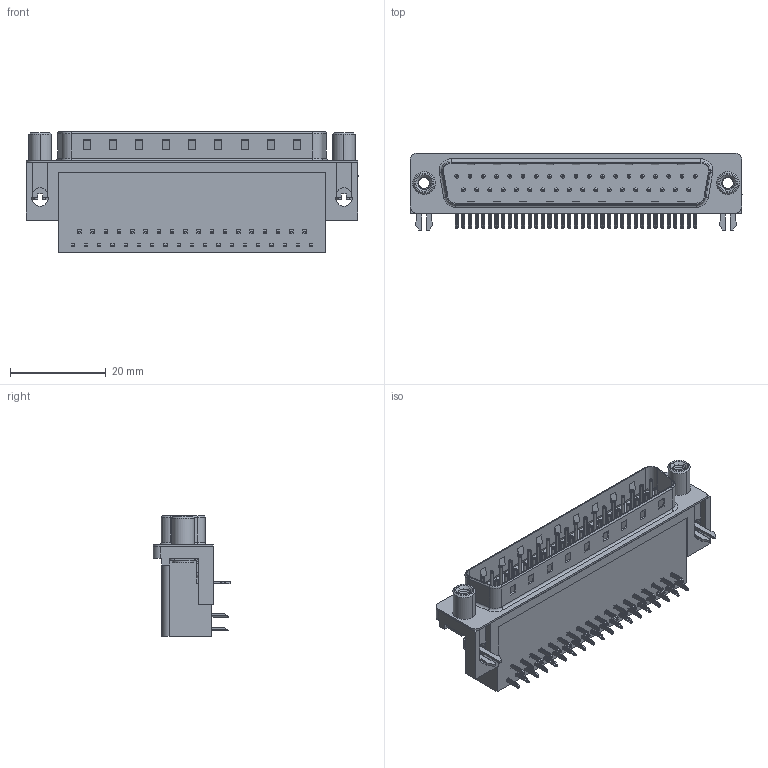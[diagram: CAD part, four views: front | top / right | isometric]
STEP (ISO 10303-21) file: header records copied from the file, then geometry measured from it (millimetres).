
FILE_DESCRIPTION (( 'STEP AP203' ), '1' );
FILE_NAME ('625-037-362-530.STEP', '2018-11-06T05:58:14', ( '' ), ( '' ), 'SwSTEP 2.0', 'SolidWorks 2016', '' );
FILE_SCHEMA (( 'CONFIG_CONTROL_DESIGN' ));
Length unit declared in the file: millimetre
Products named in the file (7): 625 Housing_37 Socket; 625 Shell_37 Socket; 625 Contact Bottom; 625 Contact Top; 625 2 Prong Board Lock; 625 Round Threaded Standoff; 625-037-362-530
Assembly tree (43 placements, depth 2):
  625-037-362-530
    625 Housing_37 Socket
    625 Shell_37 Socket
    625 Contact Bottom  x18
    625 Contact Top  x19
    625 2 Prong Board Lock  x2
    625 Round Threaded Standoff  x2
Bounding box: 69.4 x 16.25 x 25.16 mm (x, y, z)
Volume: 12689.9 mm3; surface area: 11959.2 mm2
Topology: 43 solids, 43 shells, 3235 faces, 8029 edges, 4959 vertices
Faces by surface type: plane 2037, cylinder 933, torus 237, bspline 16, cone 12
Entity records: 27659 total; most frequent: CARTESIAN_POINT 6139, DIRECTION 4128, ORIENTED_EDGE 4028, EDGE_CURVE 2014, VECTOR 1460, LINE 1460, AXIS2_PLACEMENT_3D 1334, VERTEX_POINT 1301
